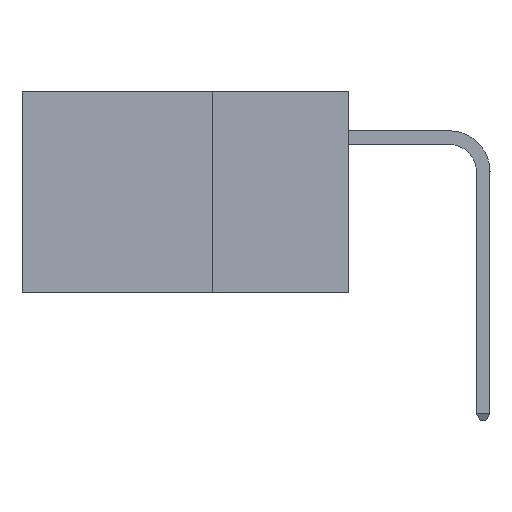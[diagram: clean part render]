
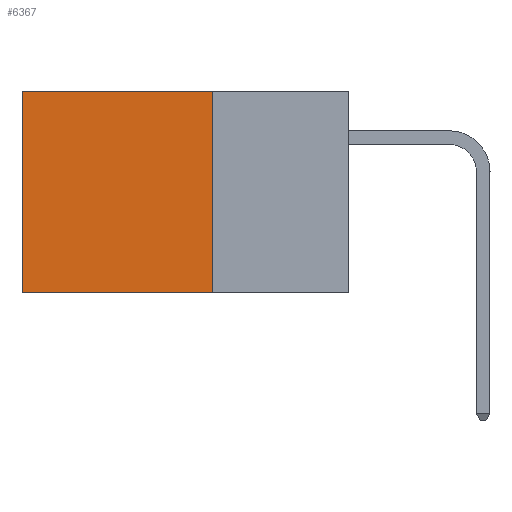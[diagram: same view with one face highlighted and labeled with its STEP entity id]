
A CAD part, left-side view. The second image highlights one B-rep face of the part: STEP entity #6367.
In plain terms, the highlighted planar face has unit normal (-1, 0, 0).
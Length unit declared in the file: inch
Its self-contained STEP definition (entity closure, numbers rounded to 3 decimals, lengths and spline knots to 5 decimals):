
#92 = EDGE_CURVE ( 'NONE', #9134, #3904, #2265, .T. ) ;
#475 = AXIS2_PLACEMENT_3D ( 'NONE', #4404, #10225, #6060 ) ;
#1475 = CARTESIAN_POINT ( 'NONE',  ( 0.2875, 0.6, -0.37 ) ) ;
#2247 = VECTOR ( 'NONE', #3522, 39.37008 ) ;
#2265 = LINE ( 'NONE', #3979, #2247 ) ;
#2661 = VECTOR ( 'NONE', #6118, 39.37008 ) ;
#2688 = LINE ( 'NONE', #6138, #2661 ) ;
#2866 = VECTOR ( 'NONE', #6140, 39.37008 ) ;
#2911 = LINE ( 'NONE', #6396, #2866 ) ;
#3265 = VECTOR ( 'NONE', #6594, 39.37008 ) ;
#3362 = LINE ( 'NONE', #6635, #3265 ) ;
#3522 = DIRECTION ( 'NONE',  ( 0., 1., 0. ) ) ;
#3723 = EDGE_CURVE ( 'NONE', #9134, #5129, #3362, .T. ) ;
#3783 = EDGE_CURVE ( 'NONE', #3904, #6486, #2911, .T. ) ;
#3784 = EDGE_CURVE ( 'NONE', #5129, #6486, #2688, .T. ) ;
#3867 = FACE_OUTER_BOUND ( 'NONE', #7489, .T. ) ;
#3904 = VERTEX_POINT ( 'NONE', #5358 ) ;
#3979 = CARTESIAN_POINT ( 'NONE',  ( 0.2875, 0.25, 0. ) ) ;
#4404 = CARTESIAN_POINT ( 'NONE',  ( 0.2875, 0.25, 0. ) ) ;
#5129 = VERTEX_POINT ( 'NONE', #10166 ) ;
#5358 = CARTESIAN_POINT ( 'NONE',  ( 0.2875, 0.6, 0. ) ) ;
#6060 = DIRECTION ( 'NONE',  ( 0., 0., -1. ) ) ;
#6118 = DIRECTION ( 'NONE',  ( 0., 1., 0. ) ) ;
#6138 = CARTESIAN_POINT ( 'NONE',  ( 0.2875, 0.25, -0.37 ) ) ;
#6140 = DIRECTION ( 'NONE',  ( 0., 0., -1. ) ) ;
#6367 = ADVANCED_FACE ( 'NONE', ( #3867 ), #9665, .F. ) ;
#6396 = CARTESIAN_POINT ( 'NONE',  ( 0.2875, 0.6, 0. ) ) ;
#6486 = VERTEX_POINT ( 'NONE', #1475 ) ;
#6594 = DIRECTION ( 'NONE',  ( 0., 0., -1. ) ) ;
#6635 = CARTESIAN_POINT ( 'NONE',  ( 0.2875, 0.25, 0. ) ) ;
#7489 = EDGE_LOOP ( 'NONE', ( #8143, #8205, #8467, #8585 ) ) ;
#8143 = ORIENTED_EDGE ( 'NONE', *, *, #3783, .T. ) ;
#8205 = ORIENTED_EDGE ( 'NONE', *, *, #3784, .F. ) ;
#8467 = ORIENTED_EDGE ( 'NONE', *, *, #3723, .F. ) ;
#8585 = ORIENTED_EDGE ( 'NONE', *, *, #92, .T. ) ;
#9134 = VERTEX_POINT ( 'NONE', #10396 ) ;
#9665 = PLANE ( 'NONE',  #475 ) ;
#10166 = CARTESIAN_POINT ( 'NONE',  ( 0.2875, 0.25, -0.37 ) ) ;
#10225 = DIRECTION ( 'NONE',  ( 1., 0., 0. ) ) ;
#10396 = CARTESIAN_POINT ( 'NONE',  ( 0.2875, 0.25, 0. ) ) ;
